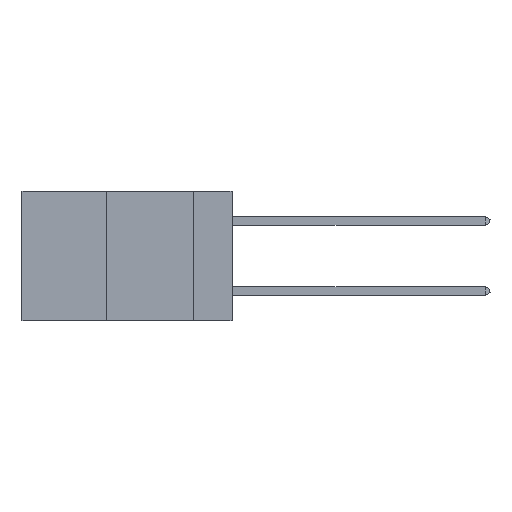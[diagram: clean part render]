
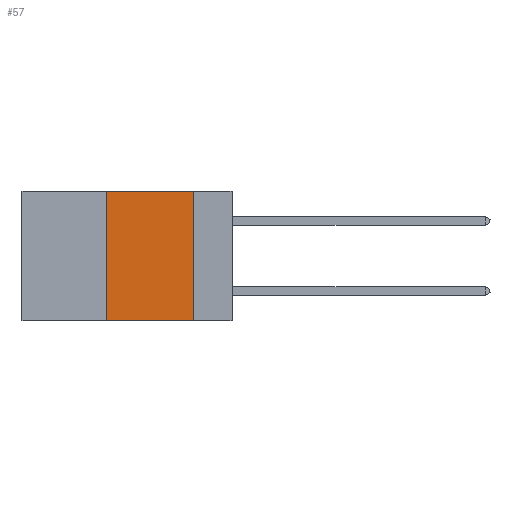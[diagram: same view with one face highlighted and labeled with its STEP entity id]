
A CAD part, left-side view. The second image highlights one B-rep face of the part: STEP entity #57.
In plain terms, the highlighted planar face has unit normal (-1, 0, 0).
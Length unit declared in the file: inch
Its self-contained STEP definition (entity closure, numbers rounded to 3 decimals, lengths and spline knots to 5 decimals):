
#57 = ADVANCED_FACE ( 'NONE', ( #28182 ), #36850, .F. ) ;
#844 = VECTOR ( 'NONE', #24915, 39.37008 ) ;
#5636 = CARTESIAN_POINT ( 'NONE',  ( 0., 0.36, 0. ) ) ;
#9472 = LINE ( 'NONE', #20065, #47535 ) ;
#11231 = CARTESIAN_POINT ( 'NONE',  ( 0., 0.6, 0. ) ) ;
#12200 = AXIS2_PLACEMENT_3D ( 'NONE', #11231, #18328, #33176 ) ;
#15334 = VECTOR ( 'NONE', #43338, 39.37008 ) ;
#16357 = CARTESIAN_POINT ( 'NONE',  ( 0., 0.36, 0. ) ) ;
#17207 = EDGE_CURVE ( 'NONE', #37343, #43732, #25187, .T. ) ;
#17444 = CARTESIAN_POINT ( 'NONE',  ( 0., 0.6, 0. ) ) ;
#17485 = EDGE_LOOP ( 'NONE', ( #27565, #22773, #27328, #19525 ) ) ;
#18328 = DIRECTION ( 'NONE',  ( 1., 0., 0. ) ) ;
#19525 = ORIENTED_EDGE ( 'NONE', *, *, #22831, .T. ) ;
#20065 = CARTESIAN_POINT ( 'NONE',  ( 0., 0.6, -0.37 ) ) ;
#20496 = LINE ( 'NONE', #17444, #844 ) ;
#22773 = ORIENTED_EDGE ( 'NONE', *, *, #45987, .F. ) ;
#22831 = EDGE_CURVE ( 'NONE', #29052, #43732, #9472, .T. ) ;
#24915 = DIRECTION ( 'NONE',  ( 0., -1., 0. ) ) ;
#25187 = LINE ( 'NONE', #36208, #15334 ) ;
#27328 = ORIENTED_EDGE ( 'NONE', *, *, #37846, .F. ) ;
#27565 = ORIENTED_EDGE ( 'NONE', *, *, #17207, .F. ) ;
#27666 = DIRECTION ( 'NONE',  ( 0., -1., 0. ) ) ;
#28182 = FACE_OUTER_BOUND ( 'NONE', #17485, .T. ) ;
#29052 = VERTEX_POINT ( 'NONE', #39798 ) ;
#30650 = VECTOR ( 'NONE', #35125, 39.37008 ) ;
#33084 = VERTEX_POINT ( 'NONE', #16357 ) ;
#33176 = DIRECTION ( 'NONE',  ( 0., 0., -1. ) ) ;
#34372 = CARTESIAN_POINT ( 'NONE',  ( 0., 0.11, -0.37 ) ) ;
#35125 = DIRECTION ( 'NONE',  ( 0., 0., 1. ) ) ;
#36208 = CARTESIAN_POINT ( 'NONE',  ( 0., 0.11, 0. ) ) ;
#36850 = PLANE ( 'NONE',  #12200 ) ;
#37343 = VERTEX_POINT ( 'NONE', #37931 ) ;
#37846 = EDGE_CURVE ( 'NONE', #29052, #33084, #46793, .T. ) ;
#37931 = CARTESIAN_POINT ( 'NONE',  ( 0., 0.11, 0. ) ) ;
#39798 = CARTESIAN_POINT ( 'NONE',  ( 0., 0.36, -0.37 ) ) ;
#43338 = DIRECTION ( 'NONE',  ( 0., 0., -1. ) ) ;
#43732 = VERTEX_POINT ( 'NONE', #34372 ) ;
#45987 = EDGE_CURVE ( 'NONE', #33084, #37343, #20496, .T. ) ;
#46793 = LINE ( 'NONE', #5636, #30650 ) ;
#47535 = VECTOR ( 'NONE', #27666, 39.37008 ) ;
